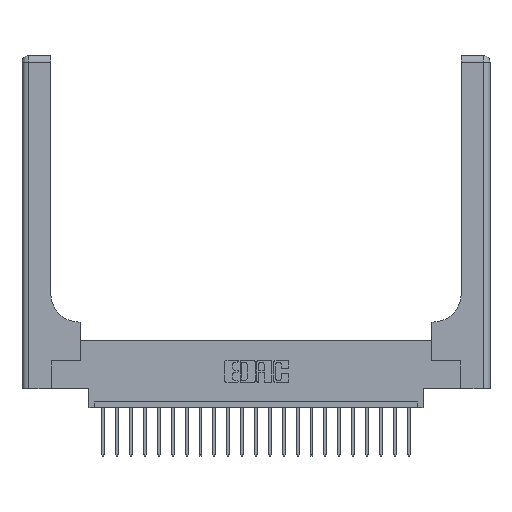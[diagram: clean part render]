
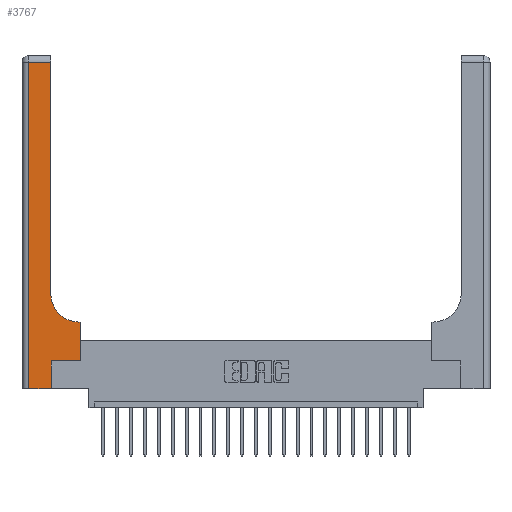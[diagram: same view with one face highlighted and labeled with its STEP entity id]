
A CAD part, top view. The second image highlights one B-rep face of the part: STEP entity #3767.
In plain terms, the highlighted planar face has unit normal (0, 0, 1).
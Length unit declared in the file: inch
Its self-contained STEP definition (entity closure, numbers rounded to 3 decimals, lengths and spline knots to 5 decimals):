
#733 = DIRECTION ( 'NONE',  ( 1., 0., 0. ) ) ;
#1312 = EDGE_CURVE ( 'NONE', #11648, #14553, #20370, .T. ) ;
#1574 = ORIENTED_EDGE ( 'NONE', *, *, #18525, .T. ) ;
#1614 = CARTESIAN_POINT ( 'NONE',  ( 0.265, 0.25, 0.37 ) ) ;
#2120 = ORIENTED_EDGE ( 'NONE', *, *, #16567, .T. ) ;
#2508 = CARTESIAN_POINT ( 'NONE',  ( 0.528, 0.6, 0.37 ) ) ;
#3016 = EDGE_CURVE ( 'NONE', #14553, #22459, #17497, .T. ) ;
#3096 = VECTOR ( 'NONE', #13544, 39.37008 ) ;
#3139 = CARTESIAN_POINT ( 'NONE',  ( 0., 2.94, 0.37 ) ) ;
#3767 = ADVANCED_FACE ( 'NONE', ( #14000 ), #20658, .F. ) ;
#3898 = CARTESIAN_POINT ( 'NONE',  ( 0.06, 0., 0.37 ) ) ;
#4048 = LINE ( 'NONE', #16388, #5963 ) ;
#4476 = VECTOR ( 'NONE', #19243, 39.37008 ) ;
#4500 = EDGE_CURVE ( 'NONE', #21682, #11849, #15297, .T. ) ;
#4612 = CARTESIAN_POINT ( 'NONE',  ( 0.26, 2.94, 0.37 ) ) ;
#4638 = LINE ( 'NONE', #3139, #8591 ) ;
#4714 = CARTESIAN_POINT ( 'NONE',  ( 0.06, 2.94, 0.37 ) ) ;
#5212 = DIRECTION ( 'NONE',  ( 0., 0., -1. ) ) ;
#5215 = LINE ( 'NONE', #20434, #3096 ) ;
#5359 = CARTESIAN_POINT ( 'NONE',  ( 0.51, 0.85, 0.37 ) ) ;
#5836 = CIRCLE ( 'NONE', #19718, 0.25 ) ;
#5963 = VECTOR ( 'NONE', #733, 39.37008 ) ;
#6840 = DIRECTION ( 'NONE',  ( 1., 0., 0. ) ) ;
#7124 = ORIENTED_EDGE ( 'NONE', *, *, #7440, .T. ) ;
#7440 = EDGE_CURVE ( 'NONE', #22194, #10088, #5215, .T. ) ;
#8022 = EDGE_CURVE ( 'NONE', #10088, #10950, #16137, .T. ) ;
#8133 = DIRECTION ( 'NONE',  ( 0., 1., 0. ) ) ;
#8591 = VECTOR ( 'NONE', #22236, 39.37008 ) ;
#9172 = CARTESIAN_POINT ( 'NONE',  ( 0., 0., 0.37 ) ) ;
#10088 = VERTEX_POINT ( 'NONE', #3898 ) ;
#10592 = EDGE_CURVE ( 'NONE', #22459, #21682, #5836, .T. ) ;
#10608 = LINE ( 'NONE', #17821, #15832 ) ;
#10816 = AXIS2_PLACEMENT_3D ( 'NONE', #12054, #5212, #15488 ) ;
#10950 = VERTEX_POINT ( 'NONE', #15714 ) ;
#11286 = ORIENTED_EDGE ( 'NONE', *, *, #16976, .T. ) ;
#11552 = CARTESIAN_POINT ( 'NONE',  ( 0.528, 0.25, 0.37 ) ) ;
#11648 = VERTEX_POINT ( 'NONE', #14543 ) ;
#11849 = VERTEX_POINT ( 'NONE', #4612 ) ;
#11933 = VERTEX_POINT ( 'NONE', #1614 ) ;
#12054 = CARTESIAN_POINT ( 'NONE',  ( 0., 3., 0.37 ) ) ;
#12317 = ORIENTED_EDGE ( 'NONE', *, *, #1312, .T. ) ;
#13343 = VECTOR ( 'NONE', #20930, 39.37008 ) ;
#13544 = DIRECTION ( 'NONE',  ( 0., -1., 0. ) ) ;
#14000 = FACE_OUTER_BOUND ( 'NONE', #18890, .T. ) ;
#14156 = DIRECTION ( 'NONE',  ( 0., 1., 0. ) ) ;
#14543 = CARTESIAN_POINT ( 'NONE',  ( 0.528, 0.25, 0.37 ) ) ;
#14553 = VERTEX_POINT ( 'NONE', #2508 ) ;
#14968 = CARTESIAN_POINT ( 'NONE',  ( 0.26, 3., 0.37 ) ) ;
#15012 = ORIENTED_EDGE ( 'NONE', *, *, #4500, .T. ) ;
#15041 = CARTESIAN_POINT ( 'NONE',  ( 0.51, 0.6, 0.37 ) ) ;
#15297 = LINE ( 'NONE', #14968, #21401 ) ;
#15488 = DIRECTION ( 'NONE',  ( -1., 0., 0. ) ) ;
#15714 = CARTESIAN_POINT ( 'NONE',  ( 0.265, 0., 0.37 ) ) ;
#15832 = VECTOR ( 'NONE', #14156, 39.37008 ) ;
#16137 = LINE ( 'NONE', #9172, #4476 ) ;
#16388 = CARTESIAN_POINT ( 'NONE',  ( 0.265, 0.25, 0.37 ) ) ;
#16567 = EDGE_CURVE ( 'NONE', #11933, #11648, #4048, .T. ) ;
#16976 = EDGE_CURVE ( 'NONE', #10950, #11933, #10608, .T. ) ;
#17497 = LINE ( 'NONE', #21272, #13343 ) ;
#17821 = CARTESIAN_POINT ( 'NONE',  ( 0.265, 0., 0.37 ) ) ;
#18525 = EDGE_CURVE ( 'NONE', #11849, #22194, #4638, .T. ) ;
#18890 = EDGE_LOOP ( 'NONE', ( #15012, #1574, #7124, #20827, #11286, #2120, #12317, #19046, #21058 ) ) ;
#19046 = ORIENTED_EDGE ( 'NONE', *, *, #3016, .T. ) ;
#19185 = DIRECTION ( 'NONE',  ( 0., 1., 0. ) ) ;
#19243 = DIRECTION ( 'NONE',  ( 1., 0., 0. ) ) ;
#19718 = AXIS2_PLACEMENT_3D ( 'NONE', #5359, #21253, #6840 ) ;
#20370 = LINE ( 'NONE', #11552, #20797 ) ;
#20434 = CARTESIAN_POINT ( 'NONE',  ( 0.06, 3., 0.37 ) ) ;
#20658 = PLANE ( 'NONE',  #10816 ) ;
#20797 = VECTOR ( 'NONE', #8133, 39.37008 ) ;
#20827 = ORIENTED_EDGE ( 'NONE', *, *, #8022, .T. ) ;
#20930 = DIRECTION ( 'NONE',  ( -1., 0., 0. ) ) ;
#21058 = ORIENTED_EDGE ( 'NONE', *, *, #10592, .T. ) ;
#21253 = DIRECTION ( 'NONE',  ( 0., 0., -1. ) ) ;
#21272 = CARTESIAN_POINT ( 'NONE',  ( 0.26, 0.6, 0.37 ) ) ;
#21401 = VECTOR ( 'NONE', #19185, 39.37008 ) ;
#21682 = VERTEX_POINT ( 'NONE', #22005 ) ;
#22005 = CARTESIAN_POINT ( 'NONE',  ( 0.26, 0.85, 0.37 ) ) ;
#22194 = VERTEX_POINT ( 'NONE', #4714 ) ;
#22236 = DIRECTION ( 'NONE',  ( -1., 0., 0. ) ) ;
#22459 = VERTEX_POINT ( 'NONE', #15041 ) ;
